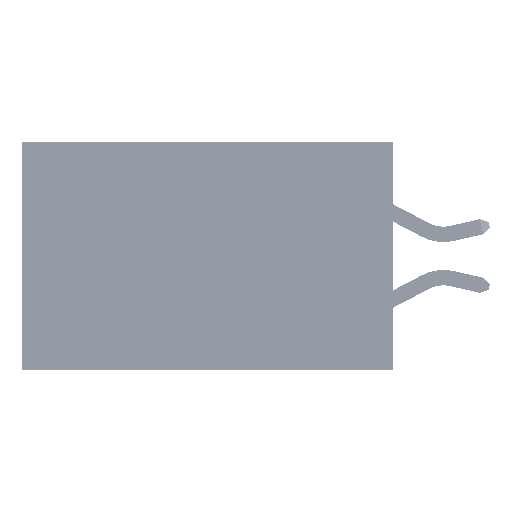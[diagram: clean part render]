
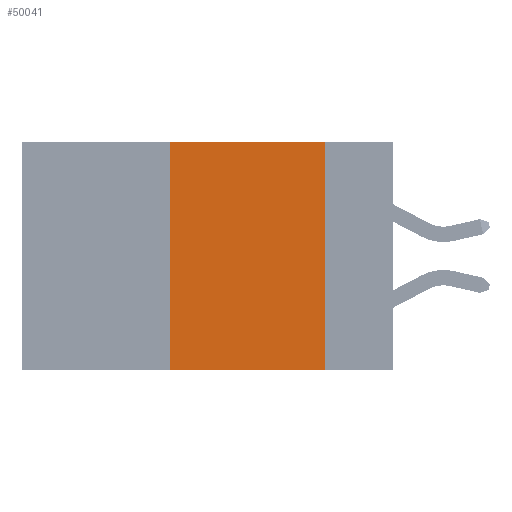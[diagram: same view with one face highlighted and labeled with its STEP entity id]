
A CAD part, left-side view. The second image highlights one B-rep face of the part: STEP entity #50041.
In plain terms, the highlighted planar face has unit normal (-1, 0, 0).
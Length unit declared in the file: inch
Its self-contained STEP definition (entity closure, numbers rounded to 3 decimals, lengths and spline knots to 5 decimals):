
#2298 = CARTESIAN_POINT ( 'NONE',  ( 0., 0.36, -0.37 ) ) ;
#3833 = CARTESIAN_POINT ( 'NONE',  ( 0., 0.11, 0. ) ) ;
#3892 = ORIENTED_EDGE ( 'NONE', *, *, #34210, .F. ) ;
#4988 = LINE ( 'NONE', #47026, #47519 ) ;
#6722 = VECTOR ( 'NONE', #7970, 39.37008 ) ;
#7970 = DIRECTION ( 'NONE',  ( 0., -1., 0. ) ) ;
#8121 = DIRECTION ( 'NONE',  ( 0., 0., -1. ) ) ;
#9172 = VECTOR ( 'NONE', #8121, 39.37008 ) ;
#9266 = VERTEX_POINT ( 'NONE', #16751 ) ;
#14273 = AXIS2_PLACEMENT_3D ( 'NONE', #32611, #40792, #16331 ) ;
#16331 = DIRECTION ( 'NONE',  ( 0., 0., -1. ) ) ;
#16751 = CARTESIAN_POINT ( 'NONE',  ( 0., 0.11, 0. ) ) ;
#17132 = ORIENTED_EDGE ( 'NONE', *, *, #32267, .F. ) ;
#17960 = LINE ( 'NONE', #36861, #6722 ) ;
#18523 = DIRECTION ( 'NONE',  ( 0., -1., 0. ) ) ;
#19402 = DIRECTION ( 'NONE',  ( 0., 0., 1. ) ) ;
#20993 = ORIENTED_EDGE ( 'NONE', *, *, #52842, .F. ) ;
#24012 = VECTOR ( 'NONE', #19402, 39.37008 ) ;
#29664 = VERTEX_POINT ( 'NONE', #50343 ) ;
#31176 = LINE ( 'NONE', #3833, #9172 ) ;
#32267 = EDGE_CURVE ( 'NONE', #9266, #29664, #31176, .T. ) ;
#32611 = CARTESIAN_POINT ( 'NONE',  ( 0., 0.6, 0. ) ) ;
#34210 = EDGE_CURVE ( 'NONE', #35494, #39329, #34882, .T. ) ;
#34882 = LINE ( 'NONE', #43687, #24012 ) ;
#35494 = VERTEX_POINT ( 'NONE', #2298 ) ;
#36703 = PLANE ( 'NONE',  #14273 ) ;
#36861 = CARTESIAN_POINT ( 'NONE',  ( 0., 0.6, 0. ) ) ;
#39329 = VERTEX_POINT ( 'NONE', #40780 ) ;
#40780 = CARTESIAN_POINT ( 'NONE',  ( 0., 0.36, 0. ) ) ;
#40792 = DIRECTION ( 'NONE',  ( 1., 0., 0. ) ) ;
#40794 = ORIENTED_EDGE ( 'NONE', *, *, #49757, .T. ) ;
#43687 = CARTESIAN_POINT ( 'NONE',  ( 0., 0.36, 0. ) ) ;
#45611 = FACE_OUTER_BOUND ( 'NONE', #52670, .T. ) ;
#47026 = CARTESIAN_POINT ( 'NONE',  ( 0., 0.6, -0.37 ) ) ;
#47519 = VECTOR ( 'NONE', #18523, 39.37008 ) ;
#49757 = EDGE_CURVE ( 'NONE', #35494, #29664, #4988, .T. ) ;
#50041 = ADVANCED_FACE ( 'NONE', ( #45611 ), #36703, .F. ) ;
#50343 = CARTESIAN_POINT ( 'NONE',  ( 0., 0.11, -0.37 ) ) ;
#52670 = EDGE_LOOP ( 'NONE', ( #17132, #20993, #3892, #40794 ) ) ;
#52842 = EDGE_CURVE ( 'NONE', #39329, #9266, #17960, .T. ) ;
